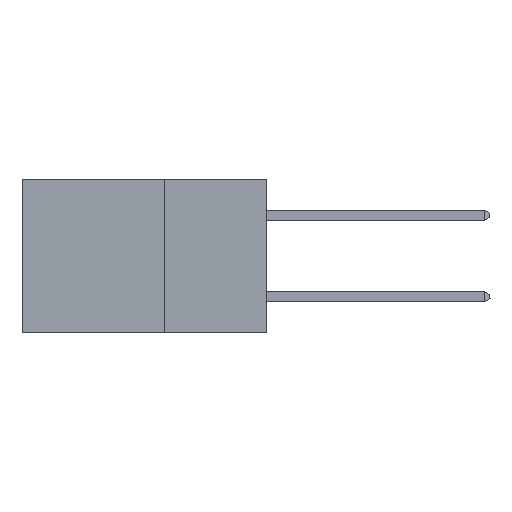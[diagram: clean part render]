
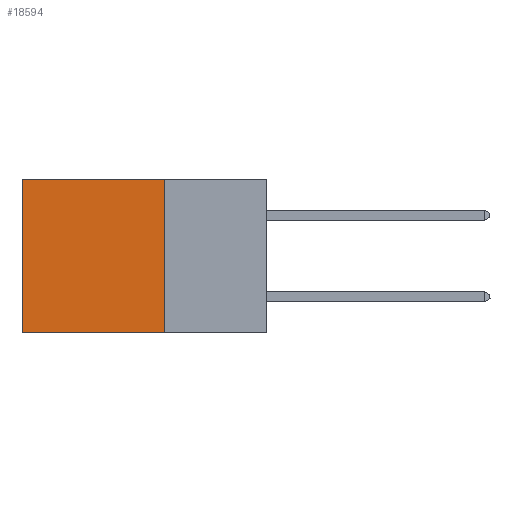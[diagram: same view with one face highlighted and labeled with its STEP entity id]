
A CAD part, left-side view. The second image highlights one B-rep face of the part: STEP entity #18594.
In plain terms, the highlighted planar face has unit normal (-1, 0, 0).
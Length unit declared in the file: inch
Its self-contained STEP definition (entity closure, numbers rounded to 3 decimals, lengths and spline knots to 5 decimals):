
#220 = VERTEX_POINT ( 'NONE', #14727 ) ;
#290 = EDGE_CURVE ( 'NONE', #17344, #19011, #14803, .T. ) ;
#670 = DIRECTION ( 'NONE',  ( 0., 0., -1. ) ) ;
#732 = CARTESIAN_POINT ( 'NONE',  ( 0.2875, 0.6, 0. ) ) ;
#1216 = VECTOR ( 'NONE', #5369, 39.37008 ) ;
#1488 = VECTOR ( 'NONE', #670, 39.37008 ) ;
#2915 = AXIS2_PLACEMENT_3D ( 'NONE', #14606, #16155, #21301 ) ;
#3232 = CARTESIAN_POINT ( 'NONE',  ( 0.2875, 0.25, 0. ) ) ;
#3533 = EDGE_CURVE ( 'NONE', #11437, #220, #10120, .T. ) ;
#3633 = CARTESIAN_POINT ( 'NONE',  ( 0.2875, 0.25, -0.375 ) ) ;
#3964 = DIRECTION ( 'NONE',  ( 0., 0., -1. ) ) ;
#5290 = ORIENTED_EDGE ( 'NONE', *, *, #15726, .T. ) ;
#5369 = DIRECTION ( 'NONE',  ( 0., 1., 0. ) ) ;
#7190 = VECTOR ( 'NONE', #3964, 39.37008 ) ;
#7274 = CARTESIAN_POINT ( 'NONE',  ( 0.2875, 0.6, -0.375 ) ) ;
#9465 = ORIENTED_EDGE ( 'NONE', *, *, #13612, .F. ) ;
#9824 = EDGE_LOOP ( 'NONE', ( #15557, #9465, #14795, #5290 ) ) ;
#10120 = LINE ( 'NONE', #7274, #7190 ) ;
#11437 = VERTEX_POINT ( 'NONE', #732 ) ;
#12992 = CARTESIAN_POINT ( 'NONE',  ( 0.2875, 0.25, -0.375 ) ) ;
#13612 = EDGE_CURVE ( 'NONE', #19011, #220, #15899, .T. ) ;
#13928 = FACE_OUTER_BOUND ( 'NONE', #9824, .T. ) ;
#14491 = DIRECTION ( 'NONE',  ( 0., 1., 0. ) ) ;
#14606 = CARTESIAN_POINT ( 'NONE',  ( 0.2875, 0.25, -0.375 ) ) ;
#14727 = CARTESIAN_POINT ( 'NONE',  ( 0.2875, 0.6, -0.375 ) ) ;
#14795 = ORIENTED_EDGE ( 'NONE', *, *, #290, .F. ) ;
#14803 = LINE ( 'NONE', #12992, #1488 ) ;
#15557 = ORIENTED_EDGE ( 'NONE', *, *, #3533, .T. ) ;
#15726 = EDGE_CURVE ( 'NONE', #17344, #11437, #17654, .T. ) ;
#15899 = LINE ( 'NONE', #21116, #21435 ) ;
#16155 = DIRECTION ( 'NONE',  ( 1., 0., 0. ) ) ;
#17344 = VERTEX_POINT ( 'NONE', #3232 ) ;
#17654 = LINE ( 'NONE', #18990, #1216 ) ;
#18594 = ADVANCED_FACE ( 'NONE', ( #13928 ), #21442, .F. ) ;
#18990 = CARTESIAN_POINT ( 'NONE',  ( 0.2875, 0.25, 0. ) ) ;
#19011 = VERTEX_POINT ( 'NONE', #3633 ) ;
#21116 = CARTESIAN_POINT ( 'NONE',  ( 0.2875, 0.25, -0.375 ) ) ;
#21301 = DIRECTION ( 'NONE',  ( 0., 0., -1. ) ) ;
#21435 = VECTOR ( 'NONE', #14491, 39.37008 ) ;
#21442 = PLANE ( 'NONE',  #2915 ) ;
